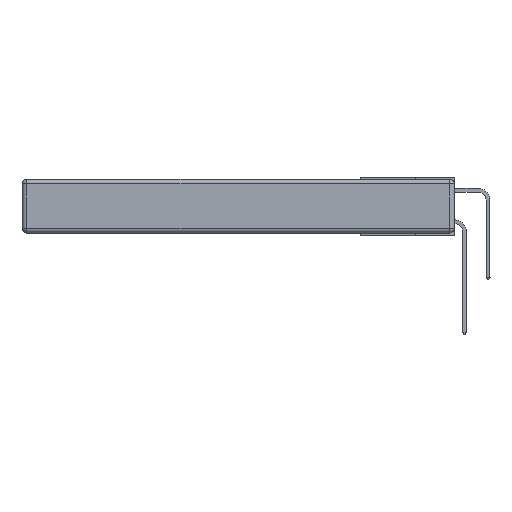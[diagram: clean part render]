
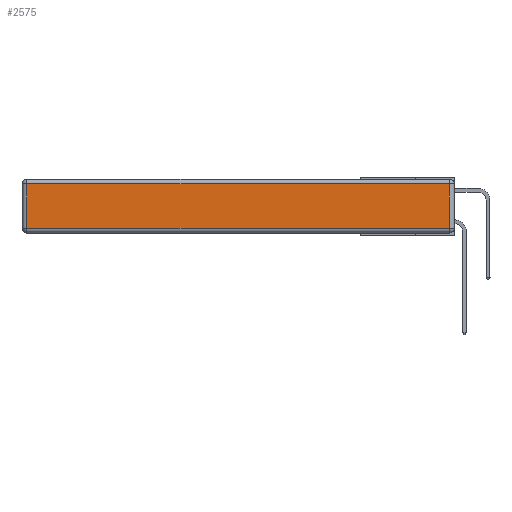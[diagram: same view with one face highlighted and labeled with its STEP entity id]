
A CAD part, left-side view. The second image highlights one B-rep face of the part: STEP entity #2575.
In plain terms, the highlighted planar face has unit normal (-1, 0, 0).
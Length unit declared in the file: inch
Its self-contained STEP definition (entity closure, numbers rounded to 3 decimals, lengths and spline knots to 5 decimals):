
#360 = EDGE_CURVE ( 'NONE', #17610, #5793, #17646, .T. ) ;
#540 = EDGE_LOOP ( 'NONE', ( #3263, #9851, #6691, #3680 ) ) ;
#1265 = VECTOR ( 'NONE', #10848, 39.37008 ) ;
#1839 = CARTESIAN_POINT ( 'NONE',  ( 0., 0.03, -0.343 ) ) ;
#2575 = ADVANCED_FACE ( 'NONE', ( #5251 ), #5432, .T. ) ;
#2826 = EDGE_CURVE ( 'NONE', #13998, #17610, #9583, .T. ) ;
#2839 = DIRECTION ( 'NONE',  ( -1., 0., 0. ) ) ;
#3263 = ORIENTED_EDGE ( 'NONE', *, *, #2826, .T. ) ;
#3680 = ORIENTED_EDGE ( 'NONE', *, *, #7589, .T. ) ;
#4129 = CARTESIAN_POINT ( 'NONE',  ( 0., 0., -0.343 ) ) ;
#4267 = DIRECTION ( 'NONE',  ( 0., 1., 0. ) ) ;
#4741 = DIRECTION ( 'NONE',  ( 0., 0., 1. ) ) ;
#5056 = LINE ( 'NONE', #8228, #7386 ) ;
#5160 = CARTESIAN_POINT ( 'NONE',  ( 0., 2.72, -0.313 ) ) ;
#5200 = VERTEX_POINT ( 'NONE', #10074 ) ;
#5251 = FACE_OUTER_BOUND ( 'NONE', #540, .T. ) ;
#5432 = PLANE ( 'NONE',  #13987 ) ;
#5793 = VERTEX_POINT ( 'NONE', #13006 ) ;
#6428 = CARTESIAN_POINT ( 'NONE',  ( 0., 2.72, -0.343 ) ) ;
#6691 = ORIENTED_EDGE ( 'NONE', *, *, #8763, .T. ) ;
#7386 = VECTOR ( 'NONE', #4267, 39.37008 ) ;
#7589 = EDGE_CURVE ( 'NONE', #5200, #13998, #8546, .T. ) ;
#8228 = CARTESIAN_POINT ( 'NONE',  ( 0., 2.75, -0.03 ) ) ;
#8546 = LINE ( 'NONE', #6428, #1265 ) ;
#8763 = EDGE_CURVE ( 'NONE', #5793, #5200, #5056, .T. ) ;
#9583 = LINE ( 'NONE', #10526, #12433 ) ;
#9851 = ORIENTED_EDGE ( 'NONE', *, *, #360, .T. ) ;
#10074 = CARTESIAN_POINT ( 'NONE',  ( 0., 2.72, -0.03 ) ) ;
#10282 = DIRECTION ( 'NONE',  ( 0., -1., 0. ) ) ;
#10526 = CARTESIAN_POINT ( 'NONE',  ( 0., 0., -0.313 ) ) ;
#10848 = DIRECTION ( 'NONE',  ( 0., 0., -1. ) ) ;
#12433 = VECTOR ( 'NONE', #10282, 39.37008 ) ;
#13006 = CARTESIAN_POINT ( 'NONE',  ( 0., 0.03, -0.03 ) ) ;
#13987 = AXIS2_PLACEMENT_3D ( 'NONE', #4129, #2839, #15015 ) ;
#13998 = VERTEX_POINT ( 'NONE', #5160 ) ;
#15015 = DIRECTION ( 'NONE',  ( 0., 0., 1. ) ) ;
#15542 = CARTESIAN_POINT ( 'NONE',  ( 0., 0.03, -0.313 ) ) ;
#16783 = VECTOR ( 'NONE', #4741, 39.37008 ) ;
#17610 = VERTEX_POINT ( 'NONE', #15542 ) ;
#17646 = LINE ( 'NONE', #1839, #16783 ) ;
